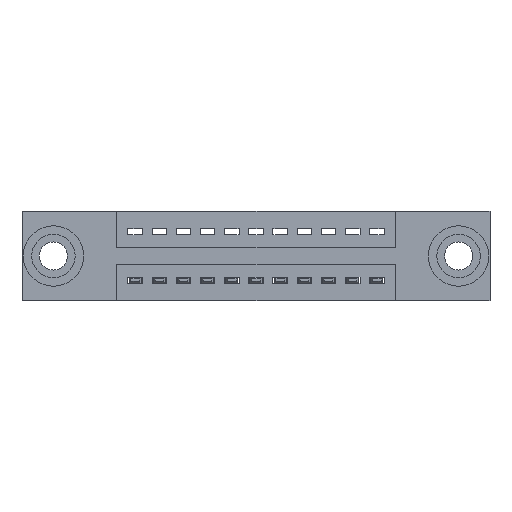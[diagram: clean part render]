
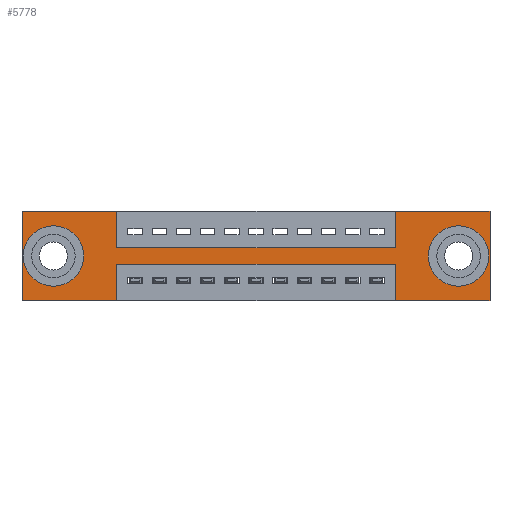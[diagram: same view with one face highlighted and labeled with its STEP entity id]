
A CAD part, front view. The second image highlights one B-rep face of the part: STEP entity #5778.
In plain terms, the highlighted planar face has unit normal (0, -1, 0).
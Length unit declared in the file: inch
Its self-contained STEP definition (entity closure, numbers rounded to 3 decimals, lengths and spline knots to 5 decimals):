
#9 = CARTESIAN_POINT ( 'NONE',  ( 0., 0., 0. ) ) ;
#56 = LINE ( 'NONE', #4158, #9750 ) ;
#96 = ORIENTED_EDGE ( 'NONE', *, *, #10159, .F. ) ;
#119 = CARTESIAN_POINT ( 'NONE',  ( 1.5425, 0., 0. ) ) ;
#424 = VERTEX_POINT ( 'NONE', #10643 ) ;
#497 = CARTESIAN_POINT ( 'NONE',  ( 0.3925, 0., -0.15 ) ) ;
#512 = LINE ( 'NONE', #8173, #2556 ) ;
#572 = DIRECTION ( 'NONE',  ( 0., 0., -1. ) ) ;
#683 = EDGE_CURVE ( 'NONE', #9537, #424, #4672, .T. ) ;
#699 = DIRECTION ( 'NONE',  ( 1., 0., 0. ) ) ;
#886 = CARTESIAN_POINT ( 'NONE',  ( 1.805, 0., -0.185 ) ) ;
#927 = FACE_BOUND ( 'NONE', #12217, .T. ) ;
#929 = ORIENTED_EDGE ( 'NONE', *, *, #8858, .F. ) ;
#952 = CARTESIAN_POINT ( 'NONE',  ( 0., 0., -0.37 ) ) ;
#1010 = ORIENTED_EDGE ( 'NONE', *, *, #7319, .F. ) ;
#1047 = LINE ( 'NONE', #4847, #4680 ) ;
#1069 = DIRECTION ( 'NONE',  ( 0., 0., -1. ) ) ;
#1099 = CARTESIAN_POINT ( 'NONE',  ( 0.13, 0., -0.107 ) ) ;
#1232 = DIRECTION ( 'NONE',  ( 0., 0., 1. ) ) ;
#1387 = AXIS2_PLACEMENT_3D ( 'NONE', #3276, #10246, #4288 ) ;
#1440 = ORIENTED_EDGE ( 'NONE', *, *, #11433, .T. ) ;
#1597 = VERTEX_POINT ( 'NONE', #3858 ) ;
#1921 = CARTESIAN_POINT ( 'NONE',  ( 0.3925, 0., -0.15 ) ) ;
#2009 = EDGE_CURVE ( 'NONE', #424, #9537, #9635, .T. ) ;
#2061 = LINE ( 'NONE', #7457, #3482 ) ;
#2082 = EDGE_LOOP ( 'NONE', ( #11558, #4097 ) ) ;
#2096 = VERTEX_POINT ( 'NONE', #6398 ) ;
#2098 = LINE ( 'NONE', #8147, #6300 ) ;
#2220 = VECTOR ( 'NONE', #6974, 39.37008 ) ;
#2556 = VECTOR ( 'NONE', #1232, 39.37008 ) ;
#2563 = ORIENTED_EDGE ( 'NONE', *, *, #9812, .F. ) ;
#2973 = VERTEX_POINT ( 'NONE', #6825 ) ;
#3222 = ORIENTED_EDGE ( 'NONE', *, *, #12443, .F. ) ;
#3276 = CARTESIAN_POINT ( 'NONE',  ( 0.13, 0., -0.185 ) ) ;
#3306 = VERTEX_POINT ( 'NONE', #4557 ) ;
#3456 = CIRCLE ( 'NONE', #1387, 0.078 ) ;
#3462 = VERTEX_POINT ( 'NONE', #12934 ) ;
#3482 = VECTOR ( 'NONE', #4490, 39.37008 ) ;
#3543 = CARTESIAN_POINT ( 'NONE',  ( 1.5425, 0., -0.22 ) ) ;
#3858 = CARTESIAN_POINT ( 'NONE',  ( 0.3925, 0., 0. ) ) ;
#3962 = EDGE_CURVE ( 'NONE', #12696, #2096, #56, .T. ) ;
#4097 = ORIENTED_EDGE ( 'NONE', *, *, #683, .T. ) ;
#4158 = CARTESIAN_POINT ( 'NONE',  ( 0.3925, 0., -0.22 ) ) ;
#4288 = DIRECTION ( 'NONE',  ( 0., 0., 1. ) ) ;
#4490 = DIRECTION ( 'NONE',  ( 0., 0., 1. ) ) ;
#4557 = CARTESIAN_POINT ( 'NONE',  ( 0., 0., -0.37 ) ) ;
#4580 = DIRECTION ( 'NONE',  ( 0., 0., 1. ) ) ;
#4672 = CIRCLE ( 'NONE', #11363, 0.078 ) ;
#4680 = VECTOR ( 'NONE', #8826, 39.37008 ) ;
#4710 = PLANE ( 'NONE',  #9585 ) ;
#4743 = ORIENTED_EDGE ( 'NONE', *, *, #6503, .F. ) ;
#4847 = CARTESIAN_POINT ( 'NONE',  ( 0.3925, 0., -0.37 ) ) ;
#4966 = DIRECTION ( 'NONE',  ( 1., 0., 0. ) ) ;
#5019 = FACE_OUTER_BOUND ( 'NONE', #7898, .T. ) ;
#5685 = CARTESIAN_POINT ( 'NONE',  ( 0., 0., -0.37 ) ) ;
#5697 = CARTESIAN_POINT ( 'NONE',  ( 1.935, 0., 0. ) ) ;
#5739 = CARTESIAN_POINT ( 'NONE',  ( 1.5425, 0., -0.37 ) ) ;
#5778 = ADVANCED_FACE ( 'NONE', ( #9697, #927, #5019 ), #4710, .T. ) ;
#6053 = CARTESIAN_POINT ( 'NONE',  ( 1.935, 0., 0. ) ) ;
#6300 = VECTOR ( 'NONE', #8997, 39.37008 ) ;
#6379 = VECTOR ( 'NONE', #572, 39.37008 ) ;
#6398 = CARTESIAN_POINT ( 'NONE',  ( 0.3925, 0., -0.22 ) ) ;
#6503 = EDGE_CURVE ( 'NONE', #12885, #8394, #12017, .T. ) ;
#6662 = DIRECTION ( 'NONE',  ( 0., -1., 0. ) ) ;
#6667 = VECTOR ( 'NONE', #1069, 39.37008 ) ;
#6825 = CARTESIAN_POINT ( 'NONE',  ( 0.3925, 0., -0.37 ) ) ;
#6974 = DIRECTION ( 'NONE',  ( 1., 0., 0. ) ) ;
#7060 = EDGE_CURVE ( 'NONE', #11871, #1597, #8077, .T. ) ;
#7156 = EDGE_CURVE ( 'NONE', #1597, #9231, #9366, .T. ) ;
#7184 = LINE ( 'NONE', #9, #2220 ) ;
#7302 = CIRCLE ( 'NONE', #10827, 0.078 ) ;
#7319 = EDGE_CURVE ( 'NONE', #2096, #2973, #1047, .T. ) ;
#7333 = VECTOR ( 'NONE', #4966, 39.37008 ) ;
#7420 = VERTEX_POINT ( 'NONE', #1099 ) ;
#7457 = CARTESIAN_POINT ( 'NONE',  ( 1.5425, 0., -0.37 ) ) ;
#7725 = CARTESIAN_POINT ( 'NONE',  ( 0.13, 0., -0.185 ) ) ;
#7898 = EDGE_LOOP ( 'NONE', ( #1010, #10449, #96, #929, #4743, #2563, #3222, #11501, #12929, #8356, #8001, #8850 ) ) ;
#8001 = ORIENTED_EDGE ( 'NONE', *, *, #9676, .F. ) ;
#8077 = LINE ( 'NONE', #10650, #9825 ) ;
#8125 = CARTESIAN_POINT ( 'NONE',  ( 1.935, 0., -0.37 ) ) ;
#8147 = CARTESIAN_POINT ( 'NONE',  ( 0., 0., -0.37 ) ) ;
#8173 = CARTESIAN_POINT ( 'NONE',  ( 0., 0., 0. ) ) ;
#8206 = CARTESIAN_POINT ( 'NONE',  ( 1.805, 0., -0.263 ) ) ;
#8267 = ORIENTED_EDGE ( 'NONE', *, *, #11353, .T. ) ;
#8274 = EDGE_CURVE ( 'NONE', #2973, #3306, #9302, .T. ) ;
#8356 = ORIENTED_EDGE ( 'NONE', *, *, #7060, .F. ) ;
#8369 = VERTEX_POINT ( 'NONE', #11015 ) ;
#8394 = VERTEX_POINT ( 'NONE', #8125 ) ;
#8508 = VECTOR ( 'NONE', #11867, 39.37008 ) ;
#8826 = DIRECTION ( 'NONE',  ( 0., 0., -1. ) ) ;
#8850 = ORIENTED_EDGE ( 'NONE', *, *, #8274, .F. ) ;
#8858 = EDGE_CURVE ( 'NONE', #8394, #12791, #2098, .T. ) ;
#8878 = VECTOR ( 'NONE', #11101, 39.37008 ) ;
#8943 = VERTEX_POINT ( 'NONE', #12616 ) ;
#8997 = DIRECTION ( 'NONE',  ( -1., 0., 0. ) ) ;
#9231 = VERTEX_POINT ( 'NONE', #497 ) ;
#9302 = LINE ( 'NONE', #952, #8508 ) ;
#9366 = LINE ( 'NONE', #10567, #6379 ) ;
#9405 = CARTESIAN_POINT ( 'NONE',  ( 0., 0., 0. ) ) ;
#9537 = VERTEX_POINT ( 'NONE', #8206 ) ;
#9585 = AXIS2_PLACEMENT_3D ( 'NONE', #5685, #6662, #12577 ) ;
#9635 = CIRCLE ( 'NONE', #9977, 0.078 ) ;
#9649 = DIRECTION ( 'NONE',  ( 0., 0., -1. ) ) ;
#9676 = EDGE_CURVE ( 'NONE', #3306, #11871, #512, .T. ) ;
#9697 = FACE_BOUND ( 'NONE', #2082, .T. ) ;
#9750 = VECTOR ( 'NONE', #11278, 39.37008 ) ;
#9760 = DIRECTION ( 'NONE',  ( 0., 1., 0. ) ) ;
#9812 = EDGE_CURVE ( 'NONE', #8943, #12885, #7184, .T. ) ;
#9825 = VECTOR ( 'NONE', #699, 39.37008 ) ;
#9977 = AXIS2_PLACEMENT_3D ( 'NONE', #11818, #12764, #9649 ) ;
#10159 = EDGE_CURVE ( 'NONE', #12791, #12696, #2061, .T. ) ;
#10246 = DIRECTION ( 'NONE',  ( 0., 1., 0. ) ) ;
#10449 = ORIENTED_EDGE ( 'NONE', *, *, #3962, .F. ) ;
#10474 = EDGE_CURVE ( 'NONE', #9231, #8369, #10635, .T. ) ;
#10567 = CARTESIAN_POINT ( 'NONE',  ( 0.3925, 0., 0. ) ) ;
#10635 = LINE ( 'NONE', #1921, #7333 ) ;
#10643 = CARTESIAN_POINT ( 'NONE',  ( 1.805, 0., -0.107 ) ) ;
#10650 = CARTESIAN_POINT ( 'NONE',  ( 0., 0., 0. ) ) ;
#10827 = AXIS2_PLACEMENT_3D ( 'NONE', #7725, #9760, #4580 ) ;
#11015 = CARTESIAN_POINT ( 'NONE',  ( 1.5425, 0., -0.15 ) ) ;
#11101 = DIRECTION ( 'NONE',  ( 0., 0., 1. ) ) ;
#11278 = DIRECTION ( 'NONE',  ( -1., 0., 0. ) ) ;
#11353 = EDGE_CURVE ( 'NONE', #7420, #3462, #3456, .T. ) ;
#11363 = AXIS2_PLACEMENT_3D ( 'NONE', #886, #11810, #11906 ) ;
#11433 = EDGE_CURVE ( 'NONE', #3462, #7420, #7302, .T. ) ;
#11501 = ORIENTED_EDGE ( 'NONE', *, *, #10474, .F. ) ;
#11558 = ORIENTED_EDGE ( 'NONE', *, *, #2009, .T. ) ;
#11810 = DIRECTION ( 'NONE',  ( 0., 1., 0. ) ) ;
#11818 = CARTESIAN_POINT ( 'NONE',  ( 1.805, 0., -0.185 ) ) ;
#11867 = DIRECTION ( 'NONE',  ( -1., 0., 0. ) ) ;
#11871 = VERTEX_POINT ( 'NONE', #9405 ) ;
#11906 = DIRECTION ( 'NONE',  ( 0., 0., -1. ) ) ;
#12016 = LINE ( 'NONE', #119, #8878 ) ;
#12017 = LINE ( 'NONE', #6053, #6667 ) ;
#12217 = EDGE_LOOP ( 'NONE', ( #8267, #1440 ) ) ;
#12443 = EDGE_CURVE ( 'NONE', #8369, #8943, #12016, .T. ) ;
#12577 = DIRECTION ( 'NONE',  ( 0., 0., -1. ) ) ;
#12616 = CARTESIAN_POINT ( 'NONE',  ( 1.5425, 0., 0. ) ) ;
#12696 = VERTEX_POINT ( 'NONE', #3543 ) ;
#12764 = DIRECTION ( 'NONE',  ( 0., 1., 0. ) ) ;
#12791 = VERTEX_POINT ( 'NONE', #5739 ) ;
#12885 = VERTEX_POINT ( 'NONE', #5697 ) ;
#12929 = ORIENTED_EDGE ( 'NONE', *, *, #7156, .F. ) ;
#12934 = CARTESIAN_POINT ( 'NONE',  ( 0.13, 0., -0.263 ) ) ;
